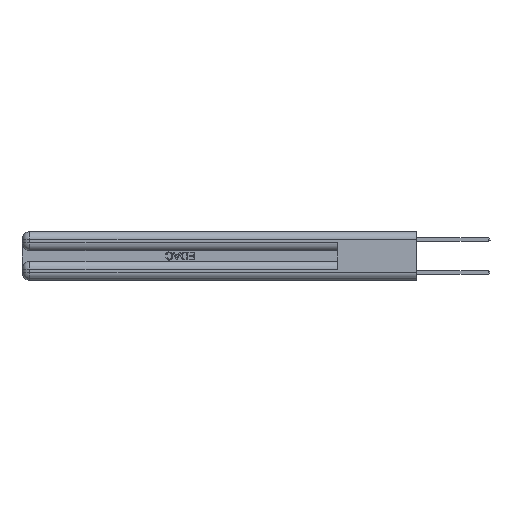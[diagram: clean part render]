
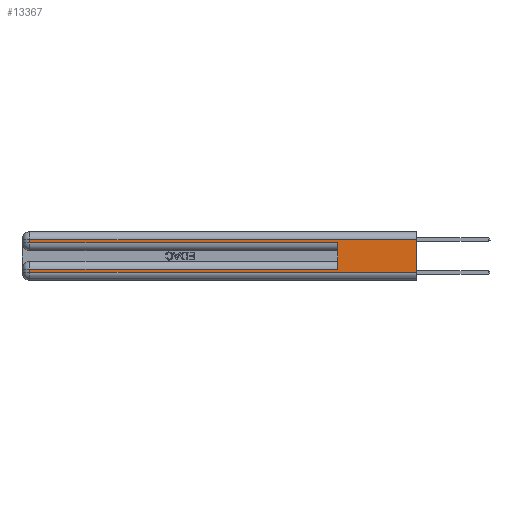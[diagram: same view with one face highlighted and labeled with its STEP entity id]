
A CAD part, left-side view. The second image highlights one B-rep face of the part: STEP entity #13367.
In plain terms, the highlighted planar face has unit normal (-1, 0, 0).
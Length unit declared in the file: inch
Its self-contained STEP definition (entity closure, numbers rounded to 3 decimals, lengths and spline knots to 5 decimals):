
#505 = VERTEX_POINT ( 'NONE', #14503 ) ;
#708 = VECTOR ( 'NONE', #11531, 39.37008 ) ;
#874 = CARTESIAN_POINT ( 'NONE',  ( 0., 0., 0.31 ) ) ;
#1036 = ORIENTED_EDGE ( 'NONE', *, *, #16605, .T. ) ;
#1591 = VECTOR ( 'NONE', #27571, 39.37008 ) ;
#1620 = LINE ( 'NONE', #2358, #7134 ) ;
#2358 = CARTESIAN_POINT ( 'NONE',  ( 0., 0.6, 0.145 ) ) ;
#2788 = DIRECTION ( 'NONE',  ( 0., 0., 1. ) ) ;
#3612 = DIRECTION ( 'NONE',  ( 1., 0., 0. ) ) ;
#3909 = ORIENTED_EDGE ( 'NONE', *, *, #5845, .T. ) ;
#4059 = DIRECTION ( 'NONE',  ( 0., 0., -1. ) ) ;
#4139 = DIRECTION ( 'NONE',  ( 0., 0., -1. ) ) ;
#4153 = CARTESIAN_POINT ( 'NONE',  ( 0., 0., 0.06 ) ) ;
#4329 = EDGE_CURVE ( 'NONE', #28582, #10517, #30881, .T. ) ;
#4864 = CARTESIAN_POINT ( 'NONE',  ( 0., 2.94, 0.37 ) ) ;
#5276 = VECTOR ( 'NONE', #10984, 39.37008 ) ;
#5291 = EDGE_CURVE ( 'NONE', #28582, #20978, #1620, .T. ) ;
#5517 = DIRECTION ( 'NONE',  ( 0., 0., -1. ) ) ;
#5845 = EDGE_CURVE ( 'NONE', #10517, #8383, #22489, .T. ) ;
#6354 = CARTESIAN_POINT ( 'NONE',  ( 0., 2.94, 0.37 ) ) ;
#6848 = CARTESIAN_POINT ( 'NONE',  ( 0., 0.6, 0.285 ) ) ;
#7134 = VECTOR ( 'NONE', #2788, 39.37008 ) ;
#7237 = EDGE_CURVE ( 'NONE', #8383, #505, #10545, .T. ) ;
#7589 = CARTESIAN_POINT ( 'NONE',  ( 0., 0., 0.37 ) ) ;
#8332 = CARTESIAN_POINT ( 'NONE',  ( 0., 0., 0.31 ) ) ;
#8383 = VERTEX_POINT ( 'NONE', #11828 ) ;
#8523 = ORIENTED_EDGE ( 'NONE', *, *, #14473, .F. ) ;
#8571 = CARTESIAN_POINT ( 'NONE',  ( 0., 0., 0.285 ) ) ;
#9165 = CARTESIAN_POINT ( 'NONE',  ( 0., 2.94, 0.31 ) ) ;
#10517 = VERTEX_POINT ( 'NONE', #26473 ) ;
#10545 = LINE ( 'NONE', #4153, #708 ) ;
#10733 = EDGE_LOOP ( 'NONE', ( #8523, #11059, #1036, #18673, #18338, #22862, #3909, #14169 ) ) ;
#10984 = DIRECTION ( 'NONE',  ( 0., 1., 0. ) ) ;
#11059 = ORIENTED_EDGE ( 'NONE', *, *, #27772, .T. ) ;
#11531 = DIRECTION ( 'NONE',  ( 0., -1., 0. ) ) ;
#11828 = CARTESIAN_POINT ( 'NONE',  ( 0., 2.94, 0.06 ) ) ;
#12259 = EDGE_CURVE ( 'NONE', #18469, #20978, #28609, .T. ) ;
#12512 = VERTEX_POINT ( 'NONE', #8332 ) ;
#13135 = DIRECTION ( 'NONE',  ( 0., -1., 0. ) ) ;
#13367 = ADVANCED_FACE ( 'NONE', ( #19494 ), #26114, .F. ) ;
#14169 = ORIENTED_EDGE ( 'NONE', *, *, #7237, .T. ) ;
#14473 = EDGE_CURVE ( 'NONE', #12512, #505, #19022, .T. ) ;
#14503 = CARTESIAN_POINT ( 'NONE',  ( 0., 0., 0.06 ) ) ;
#16605 = EDGE_CURVE ( 'NONE', #27925, #18469, #23606, .T. ) ;
#16720 = DIRECTION ( 'NONE',  ( 0., 1., 0. ) ) ;
#17697 = VECTOR ( 'NONE', #4139, 39.37008 ) ;
#17958 = VECTOR ( 'NONE', #13135, 39.37008 ) ;
#18338 = ORIENTED_EDGE ( 'NONE', *, *, #5291, .F. ) ;
#18469 = VERTEX_POINT ( 'NONE', #31058 ) ;
#18673 = ORIENTED_EDGE ( 'NONE', *, *, #12259, .T. ) ;
#19022 = LINE ( 'NONE', #7589, #31635 ) ;
#19069 = CARTESIAN_POINT ( 'NONE',  ( 0., 0., 0.085 ) ) ;
#19494 = FACE_OUTER_BOUND ( 'NONE', #10733, .T. ) ;
#20978 = VERTEX_POINT ( 'NONE', #6848 ) ;
#21044 = CARTESIAN_POINT ( 'NONE',  ( 0., 0., 0.37 ) ) ;
#21840 = LINE ( 'NONE', #874, #5276 ) ;
#21866 = AXIS2_PLACEMENT_3D ( 'NONE', #21044, #3612, #4059 ) ;
#22489 = LINE ( 'NONE', #4864, #1591 ) ;
#22862 = ORIENTED_EDGE ( 'NONE', *, *, #4329, .T. ) ;
#23606 = LINE ( 'NONE', #6354, #17697 ) ;
#24152 = VECTOR ( 'NONE', #16720, 39.37008 ) ;
#26114 = PLANE ( 'NONE',  #21866 ) ;
#26473 = CARTESIAN_POINT ( 'NONE',  ( 0., 2.94, 0.085 ) ) ;
#27571 = DIRECTION ( 'NONE',  ( 0., 0., -1. ) ) ;
#27772 = EDGE_CURVE ( 'NONE', #12512, #27925, #21840, .T. ) ;
#27925 = VERTEX_POINT ( 'NONE', #9165 ) ;
#28582 = VERTEX_POINT ( 'NONE', #31572 ) ;
#28609 = LINE ( 'NONE', #8571, #17958 ) ;
#30881 = LINE ( 'NONE', #19069, #24152 ) ;
#31058 = CARTESIAN_POINT ( 'NONE',  ( 0., 2.94, 0.285 ) ) ;
#31572 = CARTESIAN_POINT ( 'NONE',  ( 0., 0.6, 0.085 ) ) ;
#31635 = VECTOR ( 'NONE', #5517, 39.37008 ) ;
